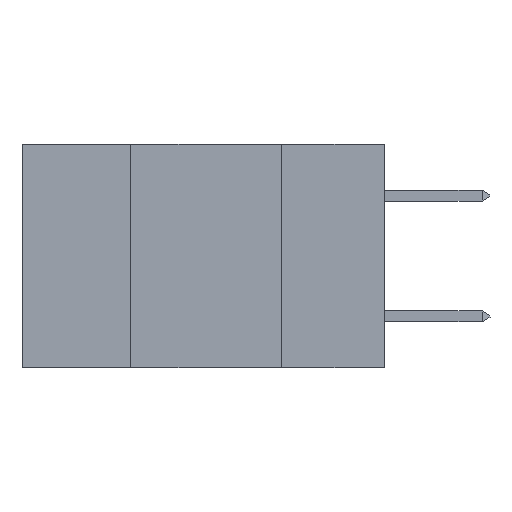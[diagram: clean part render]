
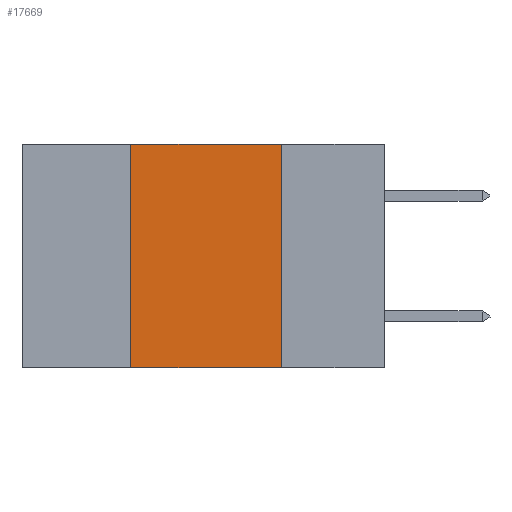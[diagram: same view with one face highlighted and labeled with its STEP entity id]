
A CAD part, left-side view. The second image highlights one B-rep face of the part: STEP entity #17669.
In plain terms, the highlighted planar face has unit normal (-1, 0, 0).
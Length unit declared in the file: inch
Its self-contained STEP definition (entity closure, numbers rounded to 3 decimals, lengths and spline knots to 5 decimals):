
#122 = EDGE_CURVE ( 'NONE', #1297, #8290, #16989, .T. ) ;
#241 = DIRECTION ( 'NONE',  ( 0., 0., -1. ) ) ;
#1011 = VECTOR ( 'NONE', #18285, 39.37008 ) ;
#1110 = EDGE_CURVE ( 'NONE', #1297, #7201, #1451, .T. ) ;
#1297 = VERTEX_POINT ( 'NONE', #4962 ) ;
#1451 = LINE ( 'NONE', #5008, #1011 ) ;
#1582 = VECTOR ( 'NONE', #2374, 39.37008 ) ;
#2160 = CARTESIAN_POINT ( 'NONE',  ( 0., 0.17, -0.37 ) ) ;
#2374 = DIRECTION ( 'NONE',  ( 0., 0., -1. ) ) ;
#2505 = LINE ( 'NONE', #9576, #17632 ) ;
#2733 = CARTESIAN_POINT ( 'NONE',  ( 0., 0.6, -0.37 ) ) ;
#2826 = EDGE_CURVE ( 'NONE', #7201, #14562, #2505, .T. ) ;
#3978 = EDGE_CURVE ( 'NONE', #14562, #8290, #9409, .T. ) ;
#4962 = CARTESIAN_POINT ( 'NONE',  ( 0., 0.42, -0.37 ) ) ;
#5008 = CARTESIAN_POINT ( 'NONE',  ( 0., 0.42, 0. ) ) ;
#5563 = CARTESIAN_POINT ( 'NONE',  ( 0., 0.17, 0. ) ) ;
#5656 = VECTOR ( 'NONE', #9401, 39.37008 ) ;
#7201 = VERTEX_POINT ( 'NONE', #8487 ) ;
#7531 = PLANE ( 'NONE',  #11808 ) ;
#7941 = ORIENTED_EDGE ( 'NONE', *, *, #1110, .F. ) ;
#8290 = VERTEX_POINT ( 'NONE', #2160 ) ;
#8487 = CARTESIAN_POINT ( 'NONE',  ( 0., 0.42, 0. ) ) ;
#8492 = FACE_OUTER_BOUND ( 'NONE', #18718, .T. ) ;
#9023 = DIRECTION ( 'NONE',  ( 1., 0., 0. ) ) ;
#9401 = DIRECTION ( 'NONE',  ( 0., -1., 0. ) ) ;
#9409 = LINE ( 'NONE', #11280, #1582 ) ;
#9497 = DIRECTION ( 'NONE',  ( 0., -1., 0. ) ) ;
#9576 = CARTESIAN_POINT ( 'NONE',  ( 0., 0.6, 0. ) ) ;
#11280 = CARTESIAN_POINT ( 'NONE',  ( 0., 0.17, 0. ) ) ;
#11808 = AXIS2_PLACEMENT_3D ( 'NONE', #17773, #9023, #241 ) ;
#11811 = ORIENTED_EDGE ( 'NONE', *, *, #122, .T. ) ;
#12240 = ORIENTED_EDGE ( 'NONE', *, *, #2826, .F. ) ;
#14562 = VERTEX_POINT ( 'NONE', #5563 ) ;
#16989 = LINE ( 'NONE', #2733, #5656 ) ;
#17632 = VECTOR ( 'NONE', #9497, 39.37008 ) ;
#17669 = ADVANCED_FACE ( 'NONE', ( #8492 ), #7531, .F. ) ;
#17773 = CARTESIAN_POINT ( 'NONE',  ( 0., 0.6, 0. ) ) ;
#18285 = DIRECTION ( 'NONE',  ( 0., 0., 1. ) ) ;
#18718 = EDGE_LOOP ( 'NONE', ( #18766, #12240, #7941, #11811 ) ) ;
#18766 = ORIENTED_EDGE ( 'NONE', *, *, #3978, .F. ) ;
